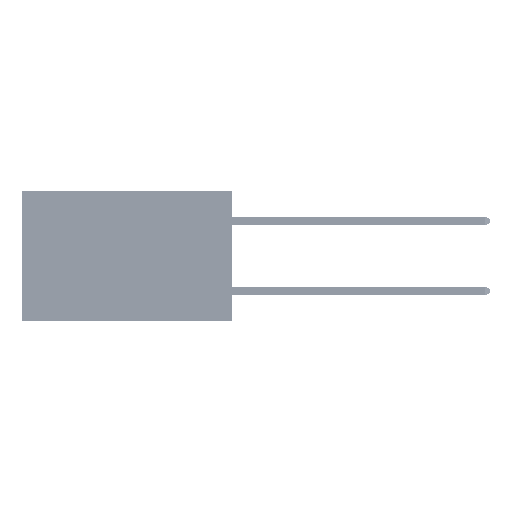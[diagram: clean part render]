
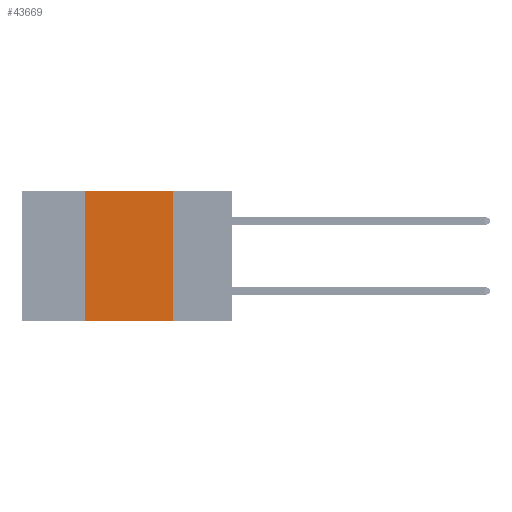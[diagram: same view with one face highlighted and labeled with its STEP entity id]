
A CAD part, left-side view. The second image highlights one B-rep face of the part: STEP entity #43669.
In plain terms, the highlighted planar face has unit normal (-1, 0, 0).
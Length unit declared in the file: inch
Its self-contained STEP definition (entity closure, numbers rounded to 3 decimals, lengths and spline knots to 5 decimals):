
#1611 = CARTESIAN_POINT ( 'NONE',  ( 0., 0.17, 0. ) ) ;
#1852 = VECTOR ( 'NONE', #2374, 39.37008 ) ;
#2118 = CARTESIAN_POINT ( 'NONE',  ( 0., 0.42, 0. ) ) ;
#2232 = VERTEX_POINT ( 'NONE', #15064 ) ;
#2374 = DIRECTION ( 'NONE',  ( 0., -1., 0. ) ) ;
#3523 = ORIENTED_EDGE ( 'NONE', *, *, #42232, .F. ) ;
#4402 = CARTESIAN_POINT ( 'NONE',  ( 0., 0.42, 0. ) ) ;
#4410 = DIRECTION ( 'NONE',  ( 1., 0., 0. ) ) ;
#5231 = LINE ( 'NONE', #1611, #27307 ) ;
#5713 = VERTEX_POINT ( 'NONE', #36329 ) ;
#7507 = LINE ( 'NONE', #4402, #35405 ) ;
#10773 = EDGE_CURVE ( 'NONE', #49925, #2232, #30738, .T. ) ;
#14584 = CARTESIAN_POINT ( 'NONE',  ( 0., 0.42, -0.37 ) ) ;
#15064 = CARTESIAN_POINT ( 'NONE',  ( 0., 0.17, -0.37 ) ) ;
#16828 = EDGE_CURVE ( 'NONE', #5713, #2232, #5231, .T. ) ;
#18222 = AXIS2_PLACEMENT_3D ( 'NONE', #30949, #4410, #46689 ) ;
#20277 = ORIENTED_EDGE ( 'NONE', *, *, #16828, .F. ) ;
#23986 = FACE_OUTER_BOUND ( 'NONE', #40414, .T. ) ;
#24298 = DIRECTION ( 'NONE',  ( 0., 0., -1. ) ) ;
#25299 = EDGE_CURVE ( 'NONE', #43280, #5713, #25839, .T. ) ;
#25839 = LINE ( 'NONE', #37941, #1852 ) ;
#25889 = ORIENTED_EDGE ( 'NONE', *, *, #25299, .F. ) ;
#27307 = VECTOR ( 'NONE', #24298, 39.37008 ) ;
#27584 = PLANE ( 'NONE',  #18222 ) ;
#30738 = LINE ( 'NONE', #43108, #47639 ) ;
#30942 = DIRECTION ( 'NONE',  ( 0., 0., 1. ) ) ;
#30949 = CARTESIAN_POINT ( 'NONE',  ( 0., 0.6, 0. ) ) ;
#34876 = DIRECTION ( 'NONE',  ( 0., -1., 0. ) ) ;
#35405 = VECTOR ( 'NONE', #30942, 39.37008 ) ;
#36329 = CARTESIAN_POINT ( 'NONE',  ( 0., 0.17, 0. ) ) ;
#37941 = CARTESIAN_POINT ( 'NONE',  ( 0., 0.6, 0. ) ) ;
#40414 = EDGE_LOOP ( 'NONE', ( #20277, #25889, #3523, #45533 ) ) ;
#42232 = EDGE_CURVE ( 'NONE', #49925, #43280, #7507, .T. ) ;
#43108 = CARTESIAN_POINT ( 'NONE',  ( 0., 0.6, -0.37 ) ) ;
#43280 = VERTEX_POINT ( 'NONE', #2118 ) ;
#43669 = ADVANCED_FACE ( 'NONE', ( #23986 ), #27584, .F. ) ;
#45533 = ORIENTED_EDGE ( 'NONE', *, *, #10773, .T. ) ;
#46689 = DIRECTION ( 'NONE',  ( 0., 0., -1. ) ) ;
#47639 = VECTOR ( 'NONE', #34876, 39.37008 ) ;
#49925 = VERTEX_POINT ( 'NONE', #14584 ) ;
